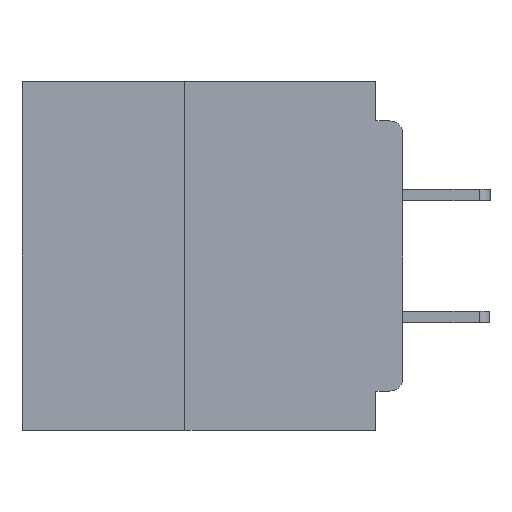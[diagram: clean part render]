
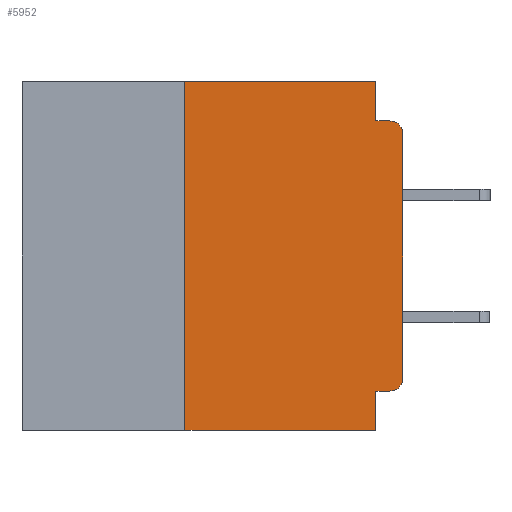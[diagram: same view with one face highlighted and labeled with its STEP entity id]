
A CAD part, left-side view. The second image highlights one B-rep face of the part: STEP entity #5952.
In plain terms, the highlighted planar face has unit normal (-1, 0, 0).
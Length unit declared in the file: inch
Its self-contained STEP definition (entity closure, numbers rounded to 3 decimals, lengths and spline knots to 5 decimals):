
#376 = PLANE ( 'NONE',  #25884 ) ;
#391 = EDGE_CURVE ( 'NONE', #22792, #19971, #1217, .T. ) ;
#655 = VERTEX_POINT ( 'NONE', #39674 ) ;
#1212 = CARTESIAN_POINT ( 'NONE',  ( 0., 0.25, 0. ) ) ;
#1217 = LINE ( 'NONE', #24599, #29343 ) ;
#1248 = CARTESIAN_POINT ( 'NONE',  ( 0., 0., -0.355 ) ) ;
#1758 = EDGE_CURVE ( 'NONE', #655, #18069, #10483, .T. ) ;
#1892 = DIRECTION ( 'NONE',  ( 0., -1., 0. ) ) ;
#2342 = VECTOR ( 'NONE', #3727, 39.37008 ) ;
#2441 = EDGE_CURVE ( 'NONE', #35197, #22792, #9874, .T. ) ;
#3134 = VECTOR ( 'NONE', #1892, 39.37008 ) ;
#3454 = LINE ( 'NONE', #17773, #2342 ) ;
#3727 = DIRECTION ( 'NONE',  ( 0., 0., 1. ) ) ;
#3798 = CARTESIAN_POINT ( 'NONE',  ( 0., 0.031, -0.4 ) ) ;
#3978 = DIRECTION ( 'NONE',  ( 0., -1., 0. ) ) ;
#4244 = LINE ( 'NONE', #43936, #3134 ) ;
#5834 = ORIENTED_EDGE ( 'NONE', *, *, #391, .F. ) ;
#5952 = ADVANCED_FACE ( 'NONE', ( #8244 ), #376, .F. ) ;
#6781 = LINE ( 'NONE', #14272, #17273 ) ;
#6819 = LINE ( 'NONE', #25985, #33761 ) ;
#8244 = FACE_OUTER_BOUND ( 'NONE', #40828, .T. ) ;
#8284 = DIRECTION ( 'NONE',  ( 0., -1., 0. ) ) ;
#8438 = ORIENTED_EDGE ( 'NONE', *, *, #32306, .F. ) ;
#9155 = DIRECTION ( 'NONE',  ( 0., 0., 1. ) ) ;
#9259 = CARTESIAN_POINT ( 'NONE',  ( 0., 0., 0. ) ) ;
#9441 = CARTESIAN_POINT ( 'NONE',  ( 0., 0.015, -0.34 ) ) ;
#9874 = LINE ( 'NONE', #37215, #27483 ) ;
#10483 = LINE ( 'NONE', #9259, #20961 ) ;
#10501 = EDGE_CURVE ( 'NONE', #42970, #655, #17090, .T. ) ;
#10957 = VERTEX_POINT ( 'NONE', #1212 ) ;
#11031 = CARTESIAN_POINT ( 'NONE',  ( 0., 0., -0.06 ) ) ;
#12334 = CARTESIAN_POINT ( 'NONE',  ( 0., 0.031, -0.045 ) ) ;
#12983 = ORIENTED_EDGE ( 'NONE', *, *, #16246, .T. ) ;
#13014 = DIRECTION ( 'NONE',  ( 0., 0., -1. ) ) ;
#13059 = VERTEX_POINT ( 'NONE', #3798 ) ;
#13288 = EDGE_CURVE ( 'NONE', #41981, #13059, #6819, .T. ) ;
#13381 = CARTESIAN_POINT ( 'NONE',  ( 0., 0.25, -0.4 ) ) ;
#13713 = EDGE_CURVE ( 'NONE', #35902, #13059, #6781, .T. ) ;
#14272 = CARTESIAN_POINT ( 'NONE',  ( 0., 0.031, -0.4 ) ) ;
#14623 = DIRECTION ( 'NONE',  ( 1., 0., 0. ) ) ;
#15473 = DIRECTION ( 'NONE',  ( 0., 1., 0. ) ) ;
#16246 = EDGE_CURVE ( 'NONE', #18069, #19971, #27852, .T. ) ;
#17090 = CIRCLE ( 'NONE', #27507, 0.015 ) ;
#17273 = VECTOR ( 'NONE', #38771, 39.37008 ) ;
#17773 = CARTESIAN_POINT ( 'NONE',  ( 0., 0.25, -0.4 ) ) ;
#18069 = VERTEX_POINT ( 'NONE', #11031 ) ;
#18291 = CARTESIAN_POINT ( 'NONE',  ( 0., 0.015, -0.06 ) ) ;
#18987 = AXIS2_PLACEMENT_3D ( 'NONE', #18291, #42760, #21845 ) ;
#19768 = ORIENTED_EDGE ( 'NONE', *, *, #10501, .T. ) ;
#19971 = VERTEX_POINT ( 'NONE', #39063 ) ;
#20961 = VECTOR ( 'NONE', #9155, 39.37008 ) ;
#21845 = DIRECTION ( 'NONE',  ( 0., 0., -1. ) ) ;
#22792 = VERTEX_POINT ( 'NONE', #12334 ) ;
#24599 = CARTESIAN_POINT ( 'NONE',  ( 0., 0., -0.045 ) ) ;
#25067 = CARTESIAN_POINT ( 'NONE',  ( 0., 0.437, 0. ) ) ;
#25738 = CARTESIAN_POINT ( 'NONE',  ( 0., 0.015, -0.355 ) ) ;
#25796 = ORIENTED_EDGE ( 'NONE', *, *, #13288, .T. ) ;
#25884 = AXIS2_PLACEMENT_3D ( 'NONE', #25067, #14623, #39110 ) ;
#25985 = CARTESIAN_POINT ( 'NONE',  ( 0., 0.437, -0.4 ) ) ;
#27483 = VECTOR ( 'NONE', #37034, 39.37008 ) ;
#27507 = AXIS2_PLACEMENT_3D ( 'NONE', #9441, #34006, #13014 ) ;
#27852 = CIRCLE ( 'NONE', #18987, 0.015 ) ;
#29343 = VECTOR ( 'NONE', #3978, 39.37008 ) ;
#32306 = EDGE_CURVE ( 'NONE', #41981, #10957, #3454, .T. ) ;
#32521 = EDGE_CURVE ( 'NONE', #42970, #35902, #40276, .T. ) ;
#33392 = ORIENTED_EDGE ( 'NONE', *, *, #32521, .F. ) ;
#33542 = ORIENTED_EDGE ( 'NONE', *, *, #1758, .T. ) ;
#33761 = VECTOR ( 'NONE', #8284, 39.37008 ) ;
#34006 = DIRECTION ( 'NONE',  ( -1., 0., 0. ) ) ;
#34333 = CARTESIAN_POINT ( 'NONE',  ( 0., 0.031, 0. ) ) ;
#34969 = ORIENTED_EDGE ( 'NONE', *, *, #13713, .F. ) ;
#35048 = EDGE_CURVE ( 'NONE', #10957, #35197, #4244, .T. ) ;
#35197 = VERTEX_POINT ( 'NONE', #34333 ) ;
#35902 = VERTEX_POINT ( 'NONE', #43307 ) ;
#37034 = DIRECTION ( 'NONE',  ( 0., 0., -1. ) ) ;
#37215 = CARTESIAN_POINT ( 'NONE',  ( 0., 0.031, 0. ) ) ;
#38771 = DIRECTION ( 'NONE',  ( 0., 0., -1. ) ) ;
#38951 = ORIENTED_EDGE ( 'NONE', *, *, #35048, .F. ) ;
#39063 = CARTESIAN_POINT ( 'NONE',  ( 0., 0.015, -0.045 ) ) ;
#39110 = DIRECTION ( 'NONE',  ( 0., 0., -1. ) ) ;
#39147 = VECTOR ( 'NONE', #15473, 39.37008 ) ;
#39674 = CARTESIAN_POINT ( 'NONE',  ( 0., 0., -0.34 ) ) ;
#40276 = LINE ( 'NONE', #1248, #39147 ) ;
#40828 = EDGE_LOOP ( 'NONE', ( #33542, #12983, #5834, #41830, #38951, #8438, #25796, #34969, #33392, #19768 ) ) ;
#41830 = ORIENTED_EDGE ( 'NONE', *, *, #2441, .F. ) ;
#41981 = VERTEX_POINT ( 'NONE', #13381 ) ;
#42760 = DIRECTION ( 'NONE',  ( -1., 0., 0. ) ) ;
#42970 = VERTEX_POINT ( 'NONE', #25738 ) ;
#43307 = CARTESIAN_POINT ( 'NONE',  ( 0., 0.031, -0.355 ) ) ;
#43936 = CARTESIAN_POINT ( 'NONE',  ( 0., 0.437, 0. ) ) ;
